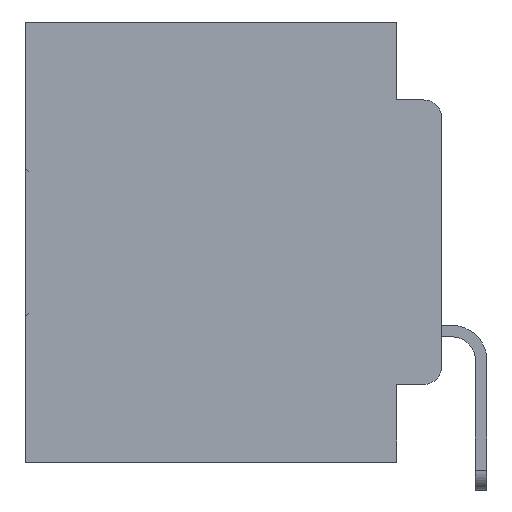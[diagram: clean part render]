
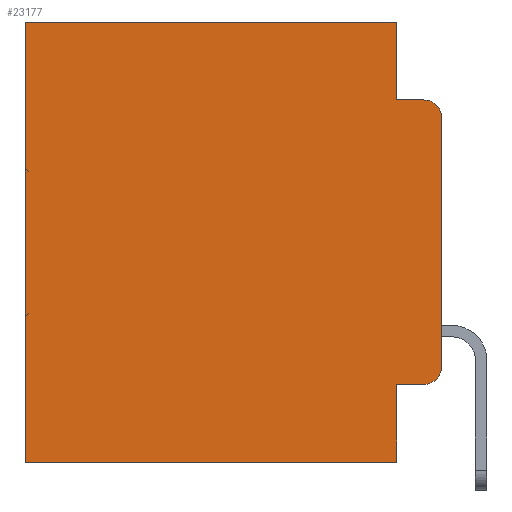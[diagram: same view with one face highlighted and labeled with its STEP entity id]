
A CAD part, left-side view. The second image highlights one B-rep face of the part: STEP entity #23177.
In plain terms, the highlighted planar face has unit normal (-1, 0, 0).
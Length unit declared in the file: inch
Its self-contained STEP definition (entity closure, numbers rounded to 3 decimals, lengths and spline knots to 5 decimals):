
#1268 = CARTESIAN_POINT ( 'NONE',  ( 0.298, 0.02, -0.3915 ) ) ;
#1415 = AXIS2_PLACEMENT_3D ( 'NONE', #1268, #19780, #4052 ) ;
#1517 = AXIS2_PLACEMENT_3D ( 'NONE', #17748, #4648, #22833 ) ;
#1606 = EDGE_CURVE ( 'NONE', #8962, #14900, #13838, .T. ) ;
#1752 = DIRECTION ( 'NONE',  ( 0., 1., 0. ) ) ;
#1922 = CIRCLE ( 'NONE', #1415, 0.02 ) ;
#3885 = FACE_OUTER_BOUND ( 'NONE', #11845, .T. ) ;
#4052 = DIRECTION ( 'NONE',  ( 0., 0., -1. ) ) ;
#4069 = VECTOR ( 'NONE', #1752, 39.37008 ) ;
#4457 = ORIENTED_EDGE ( 'NONE', *, *, #8777, .T. ) ;
#4648 = DIRECTION ( 'NONE',  ( 1., 0., 0. ) ) ;
#4883 = VERTEX_POINT ( 'NONE', #9104 ) ;
#5011 = VERTEX_POINT ( 'NONE', #6942 ) ;
#6942 = CARTESIAN_POINT ( 'NONE',  ( 0.298, 0.02, -0.0885 ) ) ;
#7037 = ORIENTED_EDGE ( 'NONE', *, *, #23754, .F. ) ;
#8188 = CARTESIAN_POINT ( 'NONE',  ( 0.298, 0.02, -0.1085 ) ) ;
#8777 = EDGE_CURVE ( 'NONE', #9029, #4883, #1922, .T. ) ;
#8876 = EDGE_CURVE ( 'NONE', #20882, #31058, #11211, .T. ) ;
#8962 = VERTEX_POINT ( 'NONE', #32302 ) ;
#9029 = VERTEX_POINT ( 'NONE', #18384 ) ;
#9104 = CARTESIAN_POINT ( 'NONE',  ( 0.298, 0., -0.3915 ) ) ;
#9109 = LINE ( 'NONE', #29141, #21928 ) ;
#9258 = EDGE_CURVE ( 'NONE', #28346, #9029, #25357, .T. ) ;
#9586 = ORIENTED_EDGE ( 'NONE', *, *, #8876, .T. ) ;
#10441 = CARTESIAN_POINT ( 'NONE',  ( 0.298, 0.473, 0. ) ) ;
#10479 = DIRECTION ( 'NONE',  ( 0., 0., -1. ) ) ;
#10781 = VECTOR ( 'NONE', #25148, 39.37008 ) ;
#10868 = DIRECTION ( 'NONE',  ( 0., 0., -1. ) ) ;
#11184 = CARTESIAN_POINT ( 'NONE',  ( 0.298, 0., -0.5 ) ) ;
#11211 = LINE ( 'NONE', #29774, #4069 ) ;
#11845 = EDGE_LOOP ( 'NONE', ( #7037, #30115, #23898, #29410, #9586, #32541, #20827, #18394, #25003, #4457 ) ) ;
#11859 = DIRECTION ( 'NONE',  ( 0., -1., 0. ) ) ;
#12371 = EDGE_CURVE ( 'NONE', #21421, #5011, #9109, .T. ) ;
#12483 = CARTESIAN_POINT ( 'NONE',  ( 0.298, 0.051, 0. ) ) ;
#12750 = CARTESIAN_POINT ( 'NONE',  ( 0.298, 0.473, -0.5 ) ) ;
#13048 = VECTOR ( 'NONE', #25539, 39.37008 ) ;
#13838 = LINE ( 'NONE', #11184, #13048 ) ;
#14088 = DIRECTION ( 'NONE',  ( 0., 0., -1. ) ) ;
#14218 = CARTESIAN_POINT ( 'NONE',  ( 0.298, 0.051, -0.4115 ) ) ;
#14647 = EDGE_CURVE ( 'NONE', #28346, #8962, #23726, .T. ) ;
#14900 = VERTEX_POINT ( 'NONE', #12750 ) ;
#15144 = PLANE ( 'NONE',  #1517 ) ;
#17603 = LINE ( 'NONE', #27433, #10781 ) ;
#17632 = EDGE_CURVE ( 'NONE', #31058, #14900, #17603, .T. ) ;
#17732 = EDGE_CURVE ( 'NONE', #20882, #21421, #21200, .T. ) ;
#17748 = CARTESIAN_POINT ( 'NONE',  ( 0.298, 0., 0. ) ) ;
#17825 = VECTOR ( 'NONE', #24583, 39.37008 ) ;
#17841 = AXIS2_PLACEMENT_3D ( 'NONE', #8188, #25903, #10868 ) ;
#18384 = CARTESIAN_POINT ( 'NONE',  ( 0.298, 0.02, -0.4115 ) ) ;
#18394 = ORIENTED_EDGE ( 'NONE', *, *, #14647, .F. ) ;
#19401 = DIRECTION ( 'NONE',  ( 0., -1., 0. ) ) ;
#19780 = DIRECTION ( 'NONE',  ( -1., 0., 0. ) ) ;
#20279 = LINE ( 'NONE', #31558, #17825 ) ;
#20438 = VECTOR ( 'NONE', #10479, 39.37008 ) ;
#20503 = VERTEX_POINT ( 'NONE', #23769 ) ;
#20827 = ORIENTED_EDGE ( 'NONE', *, *, #1606, .F. ) ;
#20882 = VERTEX_POINT ( 'NONE', #12483 ) ;
#20944 = CARTESIAN_POINT ( 'NONE',  ( 0.298, 0.051, -0.0885 ) ) ;
#21038 = CIRCLE ( 'NONE', #17841, 0.02 ) ;
#21200 = LINE ( 'NONE', #23184, #20438 ) ;
#21421 = VERTEX_POINT ( 'NONE', #20944 ) ;
#21762 = CARTESIAN_POINT ( 'NONE',  ( 0.298, 0.051, 0. ) ) ;
#21928 = VECTOR ( 'NONE', #11859, 39.37008 ) ;
#22833 = DIRECTION ( 'NONE',  ( 0., 0., -1. ) ) ;
#23177 = ADVANCED_FACE ( 'NONE', ( #3885 ), #15144, .F. ) ;
#23184 = CARTESIAN_POINT ( 'NONE',  ( 0.298, 0.051, 0. ) ) ;
#23726 = LINE ( 'NONE', #21762, #29242 ) ;
#23754 = EDGE_CURVE ( 'NONE', #20503, #4883, #20279, .T. ) ;
#23769 = CARTESIAN_POINT ( 'NONE',  ( 0.298, 0., -0.1085 ) ) ;
#23898 = ORIENTED_EDGE ( 'NONE', *, *, #12371, .F. ) ;
#24583 = DIRECTION ( 'NONE',  ( 0., 0., -1. ) ) ;
#24625 = VECTOR ( 'NONE', #19401, 39.37008 ) ;
#25003 = ORIENTED_EDGE ( 'NONE', *, *, #9258, .T. ) ;
#25148 = DIRECTION ( 'NONE',  ( 0., 0., -1. ) ) ;
#25337 = CARTESIAN_POINT ( 'NONE',  ( 0.298, 0.051, -0.4115 ) ) ;
#25357 = LINE ( 'NONE', #14218, #24625 ) ;
#25539 = DIRECTION ( 'NONE',  ( 0., 1., 0. ) ) ;
#25903 = DIRECTION ( 'NONE',  ( -1., 0., 0. ) ) ;
#27433 = CARTESIAN_POINT ( 'NONE',  ( 0.298, 0.473, 0. ) ) ;
#28346 = VERTEX_POINT ( 'NONE', #25337 ) ;
#29141 = CARTESIAN_POINT ( 'NONE',  ( 0.298, 0.051, -0.0885 ) ) ;
#29242 = VECTOR ( 'NONE', #14088, 39.37008 ) ;
#29410 = ORIENTED_EDGE ( 'NONE', *, *, #17732, .F. ) ;
#29455 = EDGE_CURVE ( 'NONE', #20503, #5011, #21038, .T. ) ;
#29774 = CARTESIAN_POINT ( 'NONE',  ( 0.298, 0., 0. ) ) ;
#30115 = ORIENTED_EDGE ( 'NONE', *, *, #29455, .T. ) ;
#31058 = VERTEX_POINT ( 'NONE', #10441 ) ;
#31558 = CARTESIAN_POINT ( 'NONE',  ( 0.298, 0., 0. ) ) ;
#32302 = CARTESIAN_POINT ( 'NONE',  ( 0.298, 0.051, -0.5 ) ) ;
#32541 = ORIENTED_EDGE ( 'NONE', *, *, #17632, .T. ) ;
